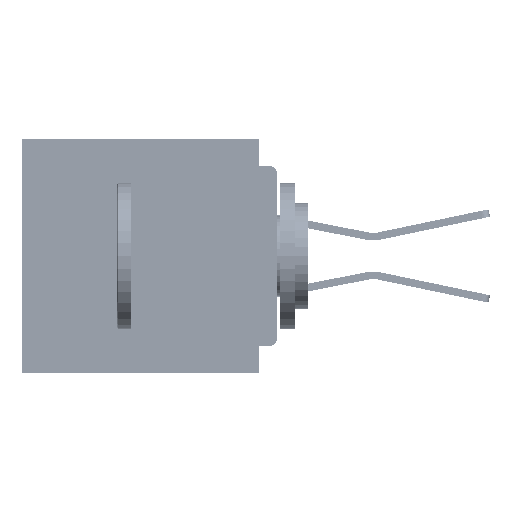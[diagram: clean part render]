
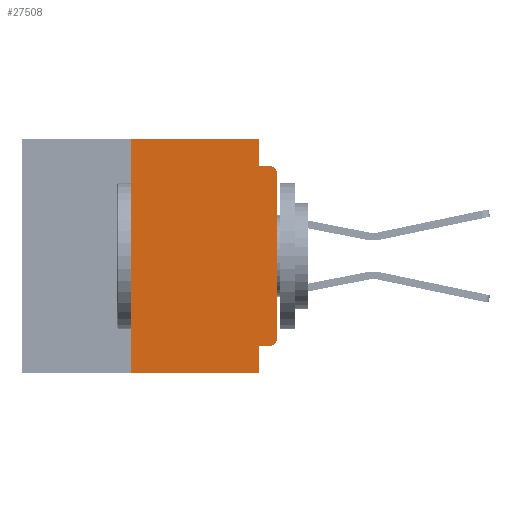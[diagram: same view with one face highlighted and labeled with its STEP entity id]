
A CAD part, left-side view. The second image highlights one B-rep face of the part: STEP entity #27508.
In plain terms, the highlighted planar face has unit normal (-1, 0, 0).
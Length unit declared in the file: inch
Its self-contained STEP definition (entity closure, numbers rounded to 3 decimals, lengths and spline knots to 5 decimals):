
#24 = EDGE_CURVE ( 'NONE', #57316, #31433, #14952, .T. ) ;
#2015 = EDGE_CURVE ( 'NONE', #57316, #2679, #2183, .T. ) ;
#2183 = LINE ( 'NONE', #25157, #17043 ) ;
#2679 = VERTEX_POINT ( 'NONE', #7263 ) ;
#3653 = EDGE_CURVE ( 'NONE', #60655, #14734, #57123, .T. ) ;
#6286 = AXIS2_PLACEMENT_3D ( 'NONE', #21821, #56134, #26798 ) ;
#6665 = AXIS2_PLACEMENT_3D ( 'NONE', #30947, #30813, #30795 ) ;
#6798 = PLANE ( 'NONE',  #6286 ) ;
#7263 = CARTESIAN_POINT ( 'NONE',  ( 0., 0.25, 0. ) ) ;
#7583 = ORIENTED_EDGE ( 'NONE', *, *, #17613, .T. ) ;
#8191 = EDGE_CURVE ( 'NONE', #45410, #9315, #51975, .T. ) ;
#9315 = VERTEX_POINT ( 'NONE', #21065 ) ;
#9397 = CARTESIAN_POINT ( 'NONE',  ( 0., 0.437, -0.4 ) ) ;
#10122 = AXIS2_PLACEMENT_3D ( 'NONE', #55940, #26607, #60838 ) ;
#10126 = LINE ( 'NONE', #32585, #60927 ) ;
#11155 = CARTESIAN_POINT ( 'NONE',  ( 0., 0.015, -0.355 ) ) ;
#12811 = CARTESIAN_POINT ( 'NONE',  ( 0., 0., -0.34 ) ) ;
#12856 = ORIENTED_EDGE ( 'NONE', *, *, #13220, .T. ) ;
#13220 = EDGE_CURVE ( 'NONE', #14734, #40091, #48578, .T. ) ;
#14734 = VERTEX_POINT ( 'NONE', #12811 ) ;
#14952 = LINE ( 'NONE', #9397, #42829 ) ;
#15370 = CARTESIAN_POINT ( 'NONE',  ( 0., 0., 0. ) ) ;
#16109 = EDGE_LOOP ( 'NONE', ( #12856, #7583, #23009, #50943, #21028, #53613, #34983, #41034, #38849, #35087 ) ) ;
#17043 = VECTOR ( 'NONE', #29260, 39.37008 ) ;
#17613 = EDGE_CURVE ( 'NONE', #40091, #22370, #27191, .T. ) ;
#20227 = VECTOR ( 'NONE', #41029, 39.37008 ) ;
#20356 = EDGE_CURVE ( 'NONE', #60655, #26123, #22158, .T. ) ;
#21028 = ORIENTED_EDGE ( 'NONE', *, *, #42078, .F. ) ;
#21065 = CARTESIAN_POINT ( 'NONE',  ( 0., 0.031, -0.045 ) ) ;
#21303 = CARTESIAN_POINT ( 'NONE',  ( 0., 0.015, -0.045 ) ) ;
#21776 = LINE ( 'NONE', #36102, #20227 ) ;
#21821 = CARTESIAN_POINT ( 'NONE',  ( 0., 0.437, 0. ) ) ;
#22010 = VECTOR ( 'NONE', #63261, 39.37008 ) ;
#22158 = LINE ( 'NONE', #55681, #46863 ) ;
#22370 = VERTEX_POINT ( 'NONE', #21303 ) ;
#23009 = ORIENTED_EDGE ( 'NONE', *, *, #23926, .F. ) ;
#23926 = EDGE_CURVE ( 'NONE', #9315, #22370, #10126, .T. ) ;
#25157 = CARTESIAN_POINT ( 'NONE',  ( 0., 0.25, -0.4 ) ) ;
#26123 = VERTEX_POINT ( 'NONE', #30134 ) ;
#26245 = CARTESIAN_POINT ( 'NONE',  ( 0., 0.25, -0.4 ) ) ;
#26336 = DIRECTION ( 'NONE',  ( 0., 1., 0. ) ) ;
#26607 = DIRECTION ( 'NONE',  ( -1., 0., 0. ) ) ;
#26798 = DIRECTION ( 'NONE',  ( 0., 0., -1. ) ) ;
#27191 = CIRCLE ( 'NONE', #10122, 0.015 ) ;
#27387 = VECTOR ( 'NONE', #31977, 39.37008 ) ;
#27508 = ADVANCED_FACE ( 'NONE', ( #31342 ), #6798, .F. ) ;
#29260 = DIRECTION ( 'NONE',  ( 0., 0., 1. ) ) ;
#30134 = CARTESIAN_POINT ( 'NONE',  ( 0., 0.031, -0.355 ) ) ;
#30795 = DIRECTION ( 'NONE',  ( 0., 0., -1. ) ) ;
#30813 = DIRECTION ( 'NONE',  ( -1., 0., 0. ) ) ;
#30947 = CARTESIAN_POINT ( 'NONE',  ( 0., 0.015, -0.34 ) ) ;
#31342 = FACE_OUTER_BOUND ( 'NONE', #16109, .T. ) ;
#31433 = VERTEX_POINT ( 'NONE', #38275 ) ;
#31977 = DIRECTION ( 'NONE',  ( 0., 0., -1. ) ) ;
#32585 = CARTESIAN_POINT ( 'NONE',  ( 0., 0., -0.045 ) ) ;
#34052 = CARTESIAN_POINT ( 'NONE',  ( 0., 0.031, -0.4 ) ) ;
#34983 = ORIENTED_EDGE ( 'NONE', *, *, #24, .T. ) ;
#35087 = ORIENTED_EDGE ( 'NONE', *, *, #3653, .T. ) ;
#36102 = CARTESIAN_POINT ( 'NONE',  ( 0., 0.437, 0. ) ) ;
#38275 = CARTESIAN_POINT ( 'NONE',  ( 0., 0.031, -0.4 ) ) ;
#38608 = VECTOR ( 'NONE', #49897, 39.37008 ) ;
#38849 = ORIENTED_EDGE ( 'NONE', *, *, #20356, .F. ) ;
#40091 = VERTEX_POINT ( 'NONE', #49198 ) ;
#41029 = DIRECTION ( 'NONE',  ( 0., -1., 0. ) ) ;
#41034 = ORIENTED_EDGE ( 'NONE', *, *, #56534, .F. ) ;
#42078 = EDGE_CURVE ( 'NONE', #2679, #45410, #21776, .T. ) ;
#42725 = DIRECTION ( 'NONE',  ( 0., -1., 0. ) ) ;
#42829 = VECTOR ( 'NONE', #56944, 39.37008 ) ;
#45410 = VERTEX_POINT ( 'NONE', #55256 ) ;
#46863 = VECTOR ( 'NONE', #26336, 39.37008 ) ;
#48578 = LINE ( 'NONE', #15370, #38608 ) ;
#49198 = CARTESIAN_POINT ( 'NONE',  ( 0., 0., -0.06 ) ) ;
#49897 = DIRECTION ( 'NONE',  ( 0., 0., 1. ) ) ;
#50943 = ORIENTED_EDGE ( 'NONE', *, *, #8191, .F. ) ;
#51975 = LINE ( 'NONE', #61286, #27387 ) ;
#53613 = ORIENTED_EDGE ( 'NONE', *, *, #2015, .F. ) ;
#55256 = CARTESIAN_POINT ( 'NONE',  ( 0., 0.031, 0. ) ) ;
#55681 = CARTESIAN_POINT ( 'NONE',  ( 0., 0., -0.355 ) ) ;
#55940 = CARTESIAN_POINT ( 'NONE',  ( 0., 0.015, -0.06 ) ) ;
#56134 = DIRECTION ( 'NONE',  ( 1., 0., 0. ) ) ;
#56534 = EDGE_CURVE ( 'NONE', #26123, #31433, #59571, .T. ) ;
#56944 = DIRECTION ( 'NONE',  ( 0., -1., 0. ) ) ;
#57123 = CIRCLE ( 'NONE', #6665, 0.015 ) ;
#57316 = VERTEX_POINT ( 'NONE', #26245 ) ;
#59571 = LINE ( 'NONE', #34052, #22010 ) ;
#60655 = VERTEX_POINT ( 'NONE', #11155 ) ;
#60838 = DIRECTION ( 'NONE',  ( 0., 0., -1. ) ) ;
#60927 = VECTOR ( 'NONE', #42725, 39.37008 ) ;
#61286 = CARTESIAN_POINT ( 'NONE',  ( 0., 0.031, 0. ) ) ;
#63261 = DIRECTION ( 'NONE',  ( 0., 0., -1. ) ) ;
